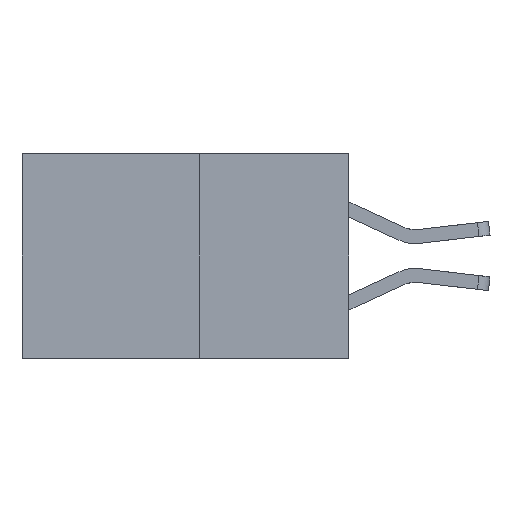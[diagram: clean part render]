
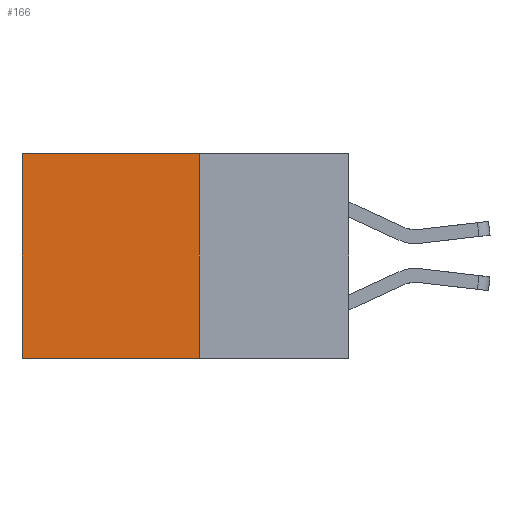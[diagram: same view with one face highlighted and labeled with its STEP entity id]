
A CAD part, left-side view. The second image highlights one B-rep face of the part: STEP entity #166.
In plain terms, the highlighted planar face has unit normal (-1, 0, 0).
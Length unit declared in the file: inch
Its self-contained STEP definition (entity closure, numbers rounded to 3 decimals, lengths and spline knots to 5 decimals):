
#14 = EDGE_CURVE ( 'NONE', #7249, #6454, #3738, .T. ) ;
#145 = EDGE_CURVE ( 'NONE', #4887, #6454, #7710, .T. ) ;
#166 = ADVANCED_FACE ( 'NONE', ( #8967 ), #1345, .F. ) ;
#877 = DIRECTION ( 'NONE',  ( 1., 0., 0. ) ) ;
#1314 = VECTOR ( 'NONE', #10004, 39.37008 ) ;
#1345 = PLANE ( 'NONE',  #5136 ) ;
#1466 = VECTOR ( 'NONE', #3608, 39.37008 ) ;
#1720 = CARTESIAN_POINT ( 'NONE',  ( 0.277, 0.59, -0.37 ) ) ;
#2405 = VERTEX_POINT ( 'NONE', #10052 ) ;
#2746 = DIRECTION ( 'NONE',  ( 0., 0., -1. ) ) ;
#2849 = EDGE_LOOP ( 'NONE', ( #4232, #3436, #6569, #3069 ) ) ;
#2908 = VECTOR ( 'NONE', #6670, 39.37008 ) ;
#3069 = ORIENTED_EDGE ( 'NONE', *, *, #3780, .T. ) ;
#3436 = ORIENTED_EDGE ( 'NONE', *, *, #14, .F. ) ;
#3608 = DIRECTION ( 'NONE',  ( 0., 1., 0. ) ) ;
#3738 = LINE ( 'NONE', #9805, #1466 ) ;
#3780 = EDGE_CURVE ( 'NONE', #2405, #4887, #4116, .T. ) ;
#3883 = VECTOR ( 'NONE', #9715, 39.37008 ) ;
#4116 = LINE ( 'NONE', #9569, #3883 ) ;
#4128 = CARTESIAN_POINT ( 'NONE',  ( 0.277, 0.59, 0. ) ) ;
#4232 = ORIENTED_EDGE ( 'NONE', *, *, #145, .T. ) ;
#4557 = CARTESIAN_POINT ( 'NONE',  ( 0.277, 0.27, -0.37 ) ) ;
#4887 = VERTEX_POINT ( 'NONE', #4128 ) ;
#4959 = LINE ( 'NONE', #6840, #2908 ) ;
#5136 = AXIS2_PLACEMENT_3D ( 'NONE', #4557, #877, #2746 ) ;
#5714 = EDGE_CURVE ( 'NONE', #2405, #7249, #4959, .T. ) ;
#5987 = CARTESIAN_POINT ( 'NONE',  ( 0.277, 0.27, -0.37 ) ) ;
#6454 = VERTEX_POINT ( 'NONE', #6627 ) ;
#6569 = ORIENTED_EDGE ( 'NONE', *, *, #5714, .F. ) ;
#6627 = CARTESIAN_POINT ( 'NONE',  ( 0.277, 0.59, -0.37 ) ) ;
#6670 = DIRECTION ( 'NONE',  ( 0., 0., -1. ) ) ;
#6840 = CARTESIAN_POINT ( 'NONE',  ( 0.277, 0.27, -0.37 ) ) ;
#7249 = VERTEX_POINT ( 'NONE', #5987 ) ;
#7710 = LINE ( 'NONE', #1720, #1314 ) ;
#8967 = FACE_OUTER_BOUND ( 'NONE', #2849, .T. ) ;
#9569 = CARTESIAN_POINT ( 'NONE',  ( 0.277, 0.27, 0. ) ) ;
#9715 = DIRECTION ( 'NONE',  ( 0., 1., 0. ) ) ;
#9805 = CARTESIAN_POINT ( 'NONE',  ( 0.277, 0.27, -0.37 ) ) ;
#10004 = DIRECTION ( 'NONE',  ( 0., 0., -1. ) ) ;
#10052 = CARTESIAN_POINT ( 'NONE',  ( 0.277, 0.27, 0. ) ) ;
